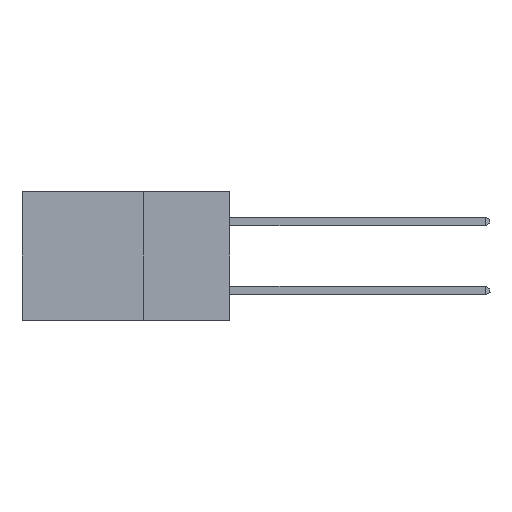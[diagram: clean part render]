
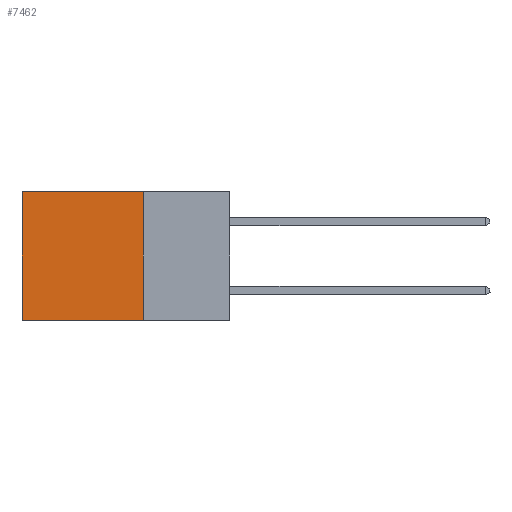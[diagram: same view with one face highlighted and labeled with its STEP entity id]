
A CAD part, left-side view. The second image highlights one B-rep face of the part: STEP entity #7462.
In plain terms, the highlighted planar face has unit normal (-1, 0, 0).
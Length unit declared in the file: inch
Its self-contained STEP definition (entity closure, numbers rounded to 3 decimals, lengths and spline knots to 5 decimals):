
#350 = CARTESIAN_POINT ( 'NONE',  ( 0.298, 0.6, 0. ) ) ;
#437 = DIRECTION ( 'NONE',  ( 0., 1., 0. ) ) ;
#843 = ORIENTED_EDGE ( 'NONE', *, *, #16330, .F. ) ;
#1422 = FACE_OUTER_BOUND ( 'NONE', #6732, .T. ) ;
#1696 = EDGE_CURVE ( 'NONE', #7195, #2015, #9760, .T. ) ;
#2015 = VERTEX_POINT ( 'NONE', #16216 ) ;
#3783 = ORIENTED_EDGE ( 'NONE', *, *, #1696, .F. ) ;
#4490 = CARTESIAN_POINT ( 'NONE',  ( 0.298, 0.25, 0. ) ) ;
#4705 = VECTOR ( 'NONE', #6538, 39.37008 ) ;
#4951 = DIRECTION ( 'NONE',  ( 0., 0., -1. ) ) ;
#5003 = CARTESIAN_POINT ( 'NONE',  ( 0.298, 0.25, 0. ) ) ;
#5745 = CARTESIAN_POINT ( 'NONE',  ( 0.298, 0.25, 0. ) ) ;
#6092 = VECTOR ( 'NONE', #11071, 39.37008 ) ;
#6250 = VECTOR ( 'NONE', #4951, 39.37008 ) ;
#6538 = DIRECTION ( 'NONE',  ( 0., 0., -1. ) ) ;
#6732 = EDGE_LOOP ( 'NONE', ( #8351, #3783, #843, #12304 ) ) ;
#7195 = VERTEX_POINT ( 'NONE', #13972 ) ;
#7462 = ADVANCED_FACE ( 'NONE', ( #1422 ), #13510, .F. ) ;
#7474 = LINE ( 'NONE', #4490, #15735 ) ;
#8351 = ORIENTED_EDGE ( 'NONE', *, *, #16937, .T. ) ;
#8640 = LINE ( 'NONE', #5003, #6250 ) ;
#9683 = LINE ( 'NONE', #14811, #4705 ) ;
#9760 = LINE ( 'NONE', #11011, #6092 ) ;
#11011 = CARTESIAN_POINT ( 'NONE',  ( 0.298, 0.25, -0.37 ) ) ;
#11071 = DIRECTION ( 'NONE',  ( 0., 1., 0. ) ) ;
#11284 = EDGE_CURVE ( 'NONE', #15652, #16294, #7474, .T. ) ;
#11951 = DIRECTION ( 'NONE',  ( 1., 0., 0. ) ) ;
#12304 = ORIENTED_EDGE ( 'NONE', *, *, #11284, .T. ) ;
#13333 = CARTESIAN_POINT ( 'NONE',  ( 0.298, 0.25, 0. ) ) ;
#13448 = DIRECTION ( 'NONE',  ( 0., 0., -1. ) ) ;
#13510 = PLANE ( 'NONE',  #15755 ) ;
#13972 = CARTESIAN_POINT ( 'NONE',  ( 0.298, 0.25, -0.37 ) ) ;
#14811 = CARTESIAN_POINT ( 'NONE',  ( 0.298, 0.6, 0. ) ) ;
#15652 = VERTEX_POINT ( 'NONE', #5745 ) ;
#15735 = VECTOR ( 'NONE', #437, 39.37008 ) ;
#15755 = AXIS2_PLACEMENT_3D ( 'NONE', #13333, #11951, #13448 ) ;
#16216 = CARTESIAN_POINT ( 'NONE',  ( 0.298, 0.6, -0.37 ) ) ;
#16294 = VERTEX_POINT ( 'NONE', #350 ) ;
#16330 = EDGE_CURVE ( 'NONE', #15652, #7195, #8640, .T. ) ;
#16937 = EDGE_CURVE ( 'NONE', #16294, #2015, #9683, .T. ) ;
